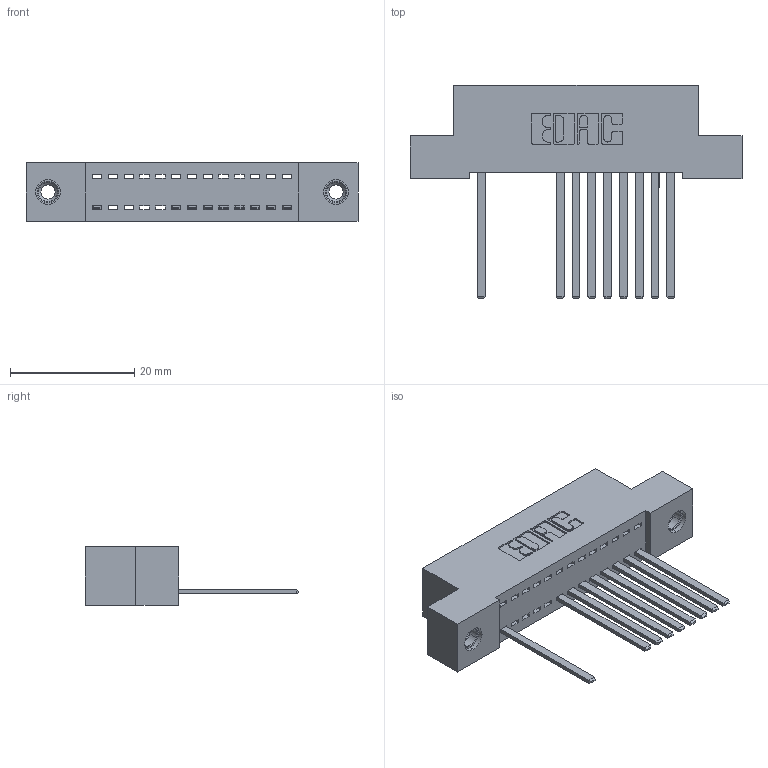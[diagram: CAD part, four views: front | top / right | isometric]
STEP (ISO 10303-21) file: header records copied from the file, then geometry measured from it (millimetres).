
FILE_DESCRIPTION (( 'STEP AP203' ), '1' );
FILE_NAME ('392-013-544-108.STEP', '2018-08-14T23:14:06', ( '' ), ( '' ), 'SwSTEP 2.0', 'SolidWorks 2016', '' );
FILE_SCHEMA (( 'CONFIG_CONTROL_DESIGN' ));
Length unit declared in the file: inch
Products named in the file (4): 345-250-001_345-250-003-102; 392-013-544-108; 342 Part_TI; 345-292-001_345-293-144
Assembly tree (12 placements, depth 2):
  392-013-544-108
    342 Part_TI
    345-292-001_345-293-144  x9
    345-250-001_345-250-003-102  x2
Bounding box: 53.34 x 34.3 x 9.4 mm (x, y, z)
Volume: 4622.8 mm3; surface area: 6324.4 mm2
Topology: 12 solids, 12 shells, 686 faces, 2025 edges, 1330 vertices
Faces by surface type: plane 488, cylinder 182, cone 12, torus 4
Entity records: 12440 total; most frequent: CARTESIAN_POINT 2148, ORIENTED_EDGE 2094, DIRECTION 1895, EDGE_CURVE 1047, VECTOR 903, LINE 903, VERTEX_POINT 692, AXIS2_PLACEMENT_3D 496
